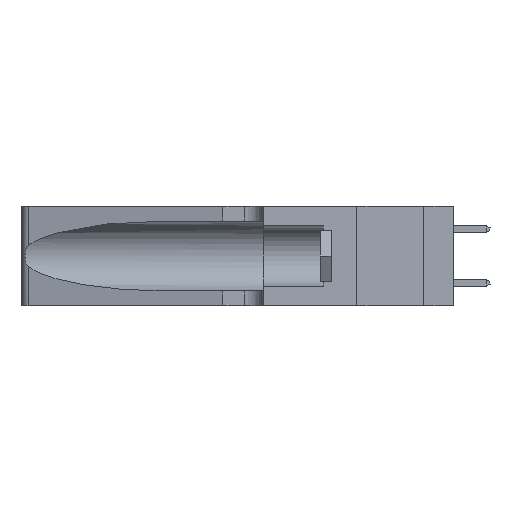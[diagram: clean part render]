
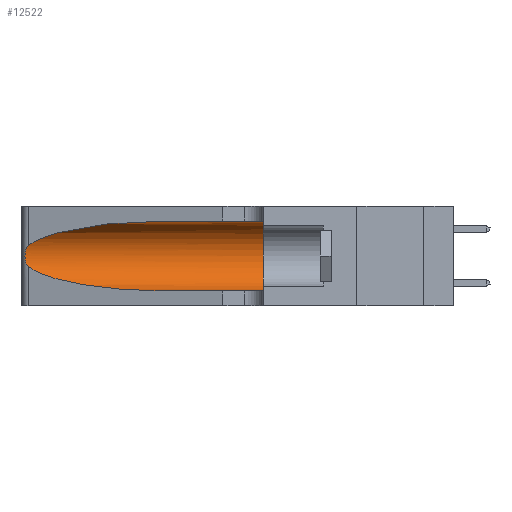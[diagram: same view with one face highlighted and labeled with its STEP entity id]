
A CAD part, left-side view. The second image highlights one B-rep face of the part: STEP entity #12522.
In plain terms, the highlighted cylindrical face has radius 3.308 mm (diameter 6.617 mm), a partial arc.
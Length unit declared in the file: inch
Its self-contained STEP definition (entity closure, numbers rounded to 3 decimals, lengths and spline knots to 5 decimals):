
#532 = CARTESIAN_POINT ( 'NONE',  ( 0.18966, 0.96281, 0.31525 ) ) ;
#1461 = ORIENTED_EDGE ( 'NONE', *, *, #6606, .F. ) ;
#1852 = LINE ( 'NONE', #30962, #16448 ) ;
#2752 = CARTESIAN_POINT ( 'NONE',  ( 0.1305, 0.72297, 0.05475 ) ) ;
#2800 = CARTESIAN_POINT ( 'NONE',  ( 0.25787, 1.23484, 0.2124 ) ) ;
#3248 = CARTESIAN_POINT ( 'NONE',  ( 0.1305, 0.72297, 0.05475 ) ) ;
#3615 = EDGE_CURVE ( 'NONE', #12657, #19411, #22564, .T. ) ;
#3791 = VECTOR ( 'NONE', #13056, 39.37008 ) ;
#5481 = CARTESIAN_POINT ( 'NONE',  ( 0.25487, 1.22718, 0.22369 ) ) ;
#5524 = CARTESIAN_POINT ( 'NONE',  ( 0.26018, 1.23835, 0.19895 ) ) ;
#5897 = DIRECTION ( 'NONE',  ( 0., 1., 0. ) ) ;
#6606 = EDGE_CURVE ( 'NONE', #10253, #11274, #14272, .T. ) ;
#7075 = CYLINDRICAL_SURFACE ( 'NONE', #10144, 0.13025 ) ;
#7328 = VERTEX_POINT ( 'NONE', #3248 ) ;
#7977 = EDGE_CURVE ( 'NONE', #19656, #12657, #9868, .T. ) ;
#8135 = CARTESIAN_POINT ( 'NONE',  ( 0.2373, 1.15595, 0.08982 ) ) ;
#8307 = CARTESIAN_POINT ( 'NONE',  ( 0.26075, 1.23896, 0.178 ) ) ;
#9150 = EDGE_LOOP ( 'NONE', ( #14744, #26175, #12062, #18250, #1461, #31351 ) ) ;
#9868 =( BOUNDED_CURVE ( )  B_SPLINE_CURVE ( 3, ( #22424, #532, #14329, #33276 ),
 .UNSPECIFIED., .F., .F. ) 
 B_SPLINE_CURVE_WITH_KNOTS ( ( 4, 4 ),
 ( 1.5708, 2.84003 ),
 .UNSPECIFIED. ) 
 CURVE ( )  GEOMETRIC_REPRESENTATION_ITEM ( )  RATIONAL_B_SPLINE_CURVE ( ( 1., 0.87, 0.87, 1. ) ) 
 REPRESENTATION_ITEM ( '' )  );
#9976 = DIRECTION ( 'NONE',  ( 0., 0., -1. ) ) ;
#10144 = AXIS2_PLACEMENT_3D ( 'NONE', #12739, #31692, #9976 ) ;
#10253 = VERTEX_POINT ( 'NONE', #10722 ) ;
#10722 = CARTESIAN_POINT ( 'NONE',  ( 0.1305, 0.35, 0.31525 ) ) ;
#11067 = CARTESIAN_POINT ( 'NONE',  ( 0.25856, 1.23593, 0.16098 ) ) ;
#11274 = VERTEX_POINT ( 'NONE', #20222 ) ;
#12062 = ORIENTED_EDGE ( 'NONE', *, *, #18405, .T. ) ;
#12522 = ADVANCED_FACE ( 'NONE', ( #16085 ), #7075, .F. ) ;
#12657 = VERTEX_POINT ( 'NONE', #32290 ) ;
#12739 = CARTESIAN_POINT ( 'NONE',  ( 0.1305, 1.61858, 0.185 ) ) ;
#13056 = DIRECTION ( 'NONE',  ( 0., -1., 0. ) ) ;
#13813 = CARTESIAN_POINT ( 'NONE',  ( 0.25639, 1.23186, 0.15144 ) ) ;
#14176 = CARTESIAN_POINT ( 'NONE',  ( 0.1305, 0.72297, 0.31525 ) ) ;
#14272 = CIRCLE ( 'NONE', #29467, 0.13025 ) ;
#14329 = CARTESIAN_POINT ( 'NONE',  ( 0.2373, 1.15595, 0.28018 ) ) ;
#14744 = ORIENTED_EDGE ( 'NONE', *, *, #7977, .T. ) ;
#14768 = DIRECTION ( 'NONE',  ( 0., -1., 0. ) ) ;
#16085 = FACE_OUTER_BOUND ( 'NONE', #9150, .T. ) ;
#16448 = VECTOR ( 'NONE', #14768, 39.37008 ) ;
#16455 = CARTESIAN_POINT ( 'NONE',  ( 0.25555, 1.22994, 0.2215 ) ) ;
#16570 = CARTESIAN_POINT ( 'NONE',  ( 0.25487, 1.22718, 0.14631 ) ) ;
#18250 = ORIENTED_EDGE ( 'NONE', *, *, #29862, .T. ) ;
#18361 = CARTESIAN_POINT ( 'NONE',  ( 0.25487, 1.22718, 0.14631 ) ) ;
#18405 = EDGE_CURVE ( 'NONE', #19411, #7328, #19970, .T. ) ;
#19135 = CARTESIAN_POINT ( 'NONE',  ( 0.18966, 0.96281, 0.05475 ) ) ;
#19183 = CARTESIAN_POINT ( 'NONE',  ( 0.25639, 1.23184, 0.21858 ) ) ;
#19411 = VERTEX_POINT ( 'NONE', #18361 ) ;
#19656 = VERTEX_POINT ( 'NONE', #14176 ) ;
#19970 =( BOUNDED_CURVE ( )  B_SPLINE_CURVE ( 3, ( #27157, #8135, #19135, #2752 ),
 .UNSPECIFIED., .F., .F. ) 
 B_SPLINE_CURVE_WITH_KNOTS ( ( 4, 4 ),
 ( 3.44316, 4.71239 ),
 .UNSPECIFIED. ) 
 CURVE ( )  GEOMETRIC_REPRESENTATION_ITEM ( )  RATIONAL_B_SPLINE_CURVE ( ( 1., 0.87, 0.87, 1. ) ) 
 REPRESENTATION_ITEM ( '' )  );
#20222 = CARTESIAN_POINT ( 'NONE',  ( 0.1305, 0.35, 0.05475 ) ) ;
#21900 = CARTESIAN_POINT ( 'NONE',  ( 0.25854, 1.2359, 0.20912 ) ) ;
#22276 = CARTESIAN_POINT ( 'NONE',  ( 0.1305, 0.35, 0.185 ) ) ;
#22424 = CARTESIAN_POINT ( 'NONE',  ( 0.1305, 0.72297, 0.31525 ) ) ;
#22564 = B_SPLINE_CURVE_WITH_KNOTS ( 'NONE', 3,
 ( #5481, #16455, #19183, #2800, #21900, #5524, #24617, #8307, #27319, #11067, #30026, #13813, #32769, #16570 ),
 .UNSPECIFIED., .F., .F.,
 ( 4, 2, 2, 2, 2, 2, 4 ),
 ( 0., 0.00027, 0.00053, 0.00107, 0.0016, 0.00187, 0.00214 ),
 .UNSPECIFIED. ) ;
#24617 = CARTESIAN_POINT ( 'NONE',  ( 0.26075, 1.23896, 0.19203 ) ) ;
#24979 = DIRECTION ( 'NONE',  ( 0., 0., 1. ) ) ;
#26175 = ORIENTED_EDGE ( 'NONE', *, *, #3615, .T. ) ;
#26281 = EDGE_CURVE ( 'NONE', #19656, #10253, #1852, .T. ) ;
#26367 = LINE ( 'NONE', #26561, #3791 ) ;
#26561 = CARTESIAN_POINT ( 'NONE',  ( 0.1305, 1.61858, 0.05475 ) ) ;
#27157 = CARTESIAN_POINT ( 'NONE',  ( 0.25487, 1.22718, 0.14631 ) ) ;
#27319 = CARTESIAN_POINT ( 'NONE',  ( 0.26017, 1.23833, 0.17102 ) ) ;
#29467 = AXIS2_PLACEMENT_3D ( 'NONE', #22276, #5897, #24979 ) ;
#29862 = EDGE_CURVE ( 'NONE', #7328, #11274, #26367, .T. ) ;
#30026 = CARTESIAN_POINT ( 'NONE',  ( 0.25789, 1.23486, 0.15765 ) ) ;
#30962 = CARTESIAN_POINT ( 'NONE',  ( 0.1305, 1.61858, 0.31525 ) ) ;
#31351 = ORIENTED_EDGE ( 'NONE', *, *, #26281, .F. ) ;
#31692 = DIRECTION ( 'NONE',  ( 0., -1., 0. ) ) ;
#32290 = CARTESIAN_POINT ( 'NONE',  ( 0.25487, 1.22718, 0.22369 ) ) ;
#32769 = CARTESIAN_POINT ( 'NONE',  ( 0.25555, 1.22993, 0.14849 ) ) ;
#33276 = CARTESIAN_POINT ( 'NONE',  ( 0.25487, 1.22718, 0.22369 ) ) ;
